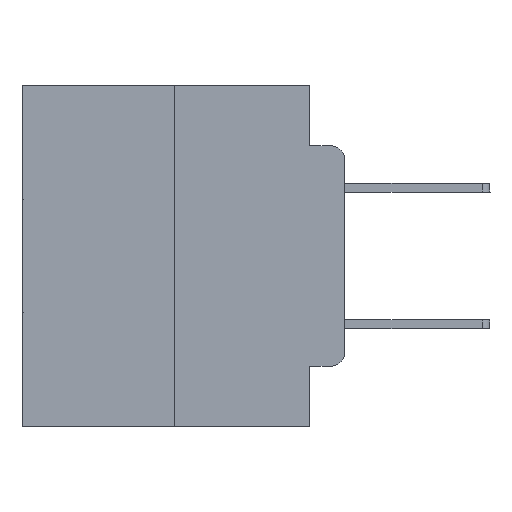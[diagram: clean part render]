
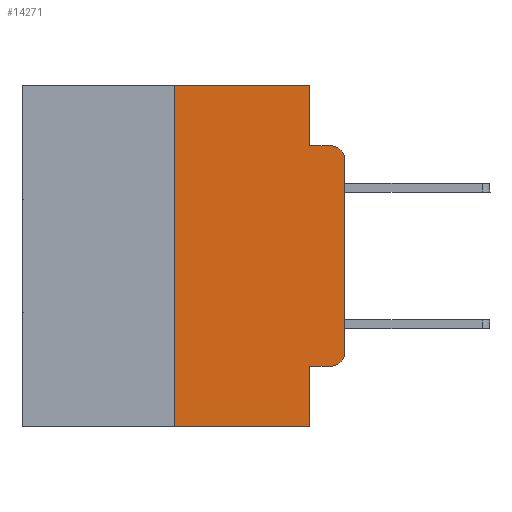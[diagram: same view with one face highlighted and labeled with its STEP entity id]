
A CAD part, left-side view. The second image highlights one B-rep face of the part: STEP entity #14271.
In plain terms, the highlighted planar face has unit normal (-1, 0, 0).
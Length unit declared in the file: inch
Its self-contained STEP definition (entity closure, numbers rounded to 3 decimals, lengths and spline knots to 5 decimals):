
#724 = VERTEX_POINT ( 'NONE', #22256 ) ;
#769 = LINE ( 'NONE', #7735, #5231 ) ;
#801 = ORIENTED_EDGE ( 'NONE', *, *, #24914, .T. ) ;
#1085 = DIRECTION ( 'NONE',  ( 0., 0., -1. ) ) ;
#1119 = ORIENTED_EDGE ( 'NONE', *, *, #6750, .T. ) ;
#2554 = DIRECTION ( 'NONE',  ( 0., 0., -1. ) ) ;
#2788 = ORIENTED_EDGE ( 'NONE', *, *, #6587, .T. ) ;
#3157 = VECTOR ( 'NONE', #25866, 39.37008 ) ;
#3273 = CARTESIAN_POINT ( 'NONE',  ( 0., 0.25, -0.5 ) ) ;
#3347 = DIRECTION ( 'NONE',  ( 0., -1., 0. ) ) ;
#4626 = VECTOR ( 'NONE', #2554, 39.37008 ) ;
#4699 = CIRCLE ( 'NONE', #22314, 0.02 ) ;
#4721 = EDGE_CURVE ( 'NONE', #20964, #17541, #10907, .T. ) ;
#5047 = CARTESIAN_POINT ( 'NONE',  ( 0., 0.051, 0. ) ) ;
#5229 = VECTOR ( 'NONE', #3347, 39.37008 ) ;
#5231 = VECTOR ( 'NONE', #10259, 39.37008 ) ;
#5365 = VECTOR ( 'NONE', #12893, 39.37008 ) ;
#5489 = VERTEX_POINT ( 'NONE', #6440 ) ;
#6032 = EDGE_CURVE ( 'NONE', #18627, #9033, #23233, .T. ) ;
#6323 = CARTESIAN_POINT ( 'NONE',  ( 0., 0.02, -0.1085 ) ) ;
#6440 = CARTESIAN_POINT ( 'NONE',  ( 0., 0.051, 0. ) ) ;
#6587 = EDGE_CURVE ( 'NONE', #18627, #8862, #769, .T. ) ;
#6599 = EDGE_LOOP ( 'NONE', ( #13362, #801, #13588, #14128, #14320, #27001, #2788, #15143, #1119, #10420 ) ) ;
#6750 = EDGE_CURVE ( 'NONE', #26508, #724, #26994, .T. ) ;
#7693 = FACE_OUTER_BOUND ( 'NONE', #6599, .T. ) ;
#7695 = CARTESIAN_POINT ( 'NONE',  ( 0., 0., -0.1085 ) ) ;
#7735 = CARTESIAN_POINT ( 'NONE',  ( 0., 0.473, -0.5 ) ) ;
#8344 = DIRECTION ( 'NONE',  ( 0., 0., 1. ) ) ;
#8736 = AXIS2_PLACEMENT_3D ( 'NONE', #9860, #27498, #1085 ) ;
#8862 = VERTEX_POINT ( 'NONE', #11711 ) ;
#9033 = VERTEX_POINT ( 'NONE', #21320 ) ;
#9860 = CARTESIAN_POINT ( 'NONE',  ( 0., 0.473, 0. ) ) ;
#10259 = DIRECTION ( 'NONE',  ( 0., -1., 0. ) ) ;
#10420 = ORIENTED_EDGE ( 'NONE', *, *, #17839, .T. ) ;
#10625 = EDGE_CURVE ( 'NONE', #5489, #20964, #26442, .T. ) ;
#10641 = CARTESIAN_POINT ( 'NONE',  ( 0., 0.051, -0.4115 ) ) ;
#10907 = LINE ( 'NONE', #17329, #5365 ) ;
#10913 = CARTESIAN_POINT ( 'NONE',  ( 0., 0., -0.3915 ) ) ;
#11109 = DIRECTION ( 'NONE',  ( 0., 0., -1. ) ) ;
#11123 = LINE ( 'NONE', #12064, #5229 ) ;
#11213 = LINE ( 'NONE', #5047, #4626 ) ;
#11711 = CARTESIAN_POINT ( 'NONE',  ( 0., 0.051, -0.5 ) ) ;
#11947 = LINE ( 'NONE', #24596, #21575 ) ;
#12064 = CARTESIAN_POINT ( 'NONE',  ( 0., 0.473, 0. ) ) ;
#12893 = DIRECTION ( 'NONE',  ( 0., -1., 0. ) ) ;
#13260 = CARTESIAN_POINT ( 'NONE',  ( 0., 0.051, 0. ) ) ;
#13362 = ORIENTED_EDGE ( 'NONE', *, *, #18376, .T. ) ;
#13588 = ORIENTED_EDGE ( 'NONE', *, *, #4721, .F. ) ;
#13768 = CARTESIAN_POINT ( 'NONE',  ( 0., 0.02, -0.3915 ) ) ;
#14128 = ORIENTED_EDGE ( 'NONE', *, *, #10625, .F. ) ;
#14271 = ADVANCED_FACE ( 'NONE', ( #7693 ), #20762, .F. ) ;
#14320 = ORIENTED_EDGE ( 'NONE', *, *, #14898, .F. ) ;
#14606 = VERTEX_POINT ( 'NONE', #10913 ) ;
#14743 = VECTOR ( 'NONE', #11109, 39.37008 ) ;
#14898 = EDGE_CURVE ( 'NONE', #9033, #5489, #11123, .T. ) ;
#15143 = ORIENTED_EDGE ( 'NONE', *, *, #19574, .F. ) ;
#15307 = CARTESIAN_POINT ( 'NONE',  ( 0., 0.02, -0.0885 ) ) ;
#15546 = CARTESIAN_POINT ( 'NONE',  ( 0., 0.051, -0.0885 ) ) ;
#16081 = DIRECTION ( 'NONE',  ( -1., 0., 0. ) ) ;
#16772 = CIRCLE ( 'NONE', #25885, 0.02 ) ;
#17329 = CARTESIAN_POINT ( 'NONE',  ( 0., 0.051, -0.0885 ) ) ;
#17409 = VECTOR ( 'NONE', #8344, 39.37008 ) ;
#17463 = DIRECTION ( 'NONE',  ( -1., 0., 0. ) ) ;
#17541 = VERTEX_POINT ( 'NONE', #15307 ) ;
#17552 = DIRECTION ( 'NONE',  ( 0., 0., -1. ) ) ;
#17839 = EDGE_CURVE ( 'NONE', #724, #14606, #4699, .T. ) ;
#18376 = EDGE_CURVE ( 'NONE', #14606, #26391, #11947, .T. ) ;
#18627 = VERTEX_POINT ( 'NONE', #3273 ) ;
#19574 = EDGE_CURVE ( 'NONE', #26508, #8862, #11213, .T. ) ;
#20196 = DIRECTION ( 'NONE',  ( 0., 0., 1. ) ) ;
#20762 = PLANE ( 'NONE',  #8736 ) ;
#20964 = VERTEX_POINT ( 'NONE', #15546 ) ;
#21320 = CARTESIAN_POINT ( 'NONE',  ( 0., 0.25, 0. ) ) ;
#21575 = VECTOR ( 'NONE', #20196, 39.37008 ) ;
#22256 = CARTESIAN_POINT ( 'NONE',  ( 0., 0.02, -0.4115 ) ) ;
#22314 = AXIS2_PLACEMENT_3D ( 'NONE', #13768, #16081, #22714 ) ;
#22714 = DIRECTION ( 'NONE',  ( 0., 0., -1. ) ) ;
#23233 = LINE ( 'NONE', #25999, #17409 ) ;
#23811 = CARTESIAN_POINT ( 'NONE',  ( 0., 0.051, -0.4115 ) ) ;
#24596 = CARTESIAN_POINT ( 'NONE',  ( 0., 0., 0. ) ) ;
#24914 = EDGE_CURVE ( 'NONE', #26391, #17541, #16772, .T. ) ;
#25866 = DIRECTION ( 'NONE',  ( 0., -1., 0. ) ) ;
#25885 = AXIS2_PLACEMENT_3D ( 'NONE', #6323, #17463, #17552 ) ;
#25999 = CARTESIAN_POINT ( 'NONE',  ( 0., 0.25, 0. ) ) ;
#26391 = VERTEX_POINT ( 'NONE', #7695 ) ;
#26442 = LINE ( 'NONE', #13260, #14743 ) ;
#26508 = VERTEX_POINT ( 'NONE', #23811 ) ;
#26994 = LINE ( 'NONE', #10641, #3157 ) ;
#27001 = ORIENTED_EDGE ( 'NONE', *, *, #6032, .F. ) ;
#27498 = DIRECTION ( 'NONE',  ( 1., 0., 0. ) ) ;
